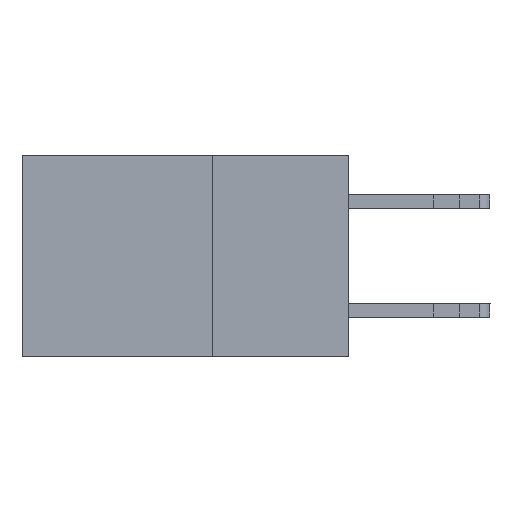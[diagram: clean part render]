
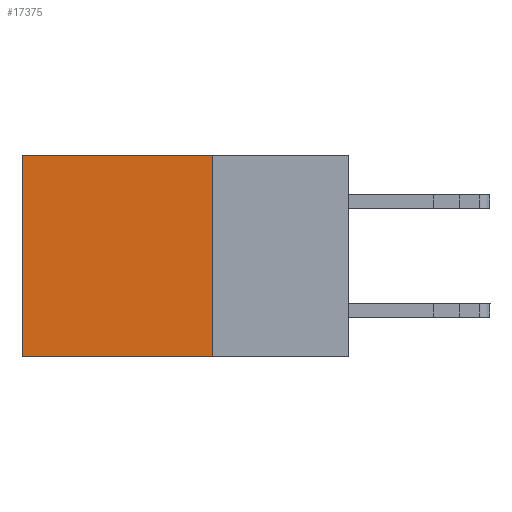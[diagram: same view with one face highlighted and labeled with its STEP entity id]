
A CAD part, left-side view. The second image highlights one B-rep face of the part: STEP entity #17375.
In plain terms, the highlighted planar face has unit normal (-1, 0, 0).
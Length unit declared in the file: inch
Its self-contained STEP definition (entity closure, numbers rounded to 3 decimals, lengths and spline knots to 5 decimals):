
#724 = VECTOR ( 'NONE', #16807, 39.37008 ) ;
#845 = DIRECTION ( 'NONE',  ( 1., 0., 0. ) ) ;
#959 = VERTEX_POINT ( 'NONE', #1659 ) ;
#1659 = CARTESIAN_POINT ( 'NONE',  ( 0.298, 0.25, 0. ) ) ;
#2360 = DIRECTION ( 'NONE',  ( 0., 0., -1. ) ) ;
#2412 = PLANE ( 'NONE',  #18329 ) ;
#2711 = DIRECTION ( 'NONE',  ( 0., 0., -1. ) ) ;
#4101 = DIRECTION ( 'NONE',  ( 0., 1., 0. ) ) ;
#4830 = ORIENTED_EDGE ( 'NONE', *, *, #10977, .T. ) ;
#5261 = CARTESIAN_POINT ( 'NONE',  ( 0.298, 0.25, 0. ) ) ;
#5357 = VECTOR ( 'NONE', #4101, 39.37008 ) ;
#6009 = EDGE_CURVE ( 'NONE', #14056, #12312, #6137, .T. ) ;
#6137 = LINE ( 'NONE', #12407, #724 ) ;
#7092 = ORIENTED_EDGE ( 'NONE', *, *, #12363, .F. ) ;
#8782 = LINE ( 'NONE', #12883, #5357 ) ;
#9106 = ORIENTED_EDGE ( 'NONE', *, *, #16862, .T. ) ;
#10977 = EDGE_CURVE ( 'NONE', #959, #15305, #8782, .T. ) ;
#12312 = VERTEX_POINT ( 'NONE', #12969 ) ;
#12363 = EDGE_CURVE ( 'NONE', #959, #14056, #14022, .T. ) ;
#12383 = CARTESIAN_POINT ( 'NONE',  ( 0.298, 0.6, 0. ) ) ;
#12407 = CARTESIAN_POINT ( 'NONE',  ( 0.298, 0.25, -0.37 ) ) ;
#12883 = CARTESIAN_POINT ( 'NONE',  ( 0.298, 0.25, 0. ) ) ;
#12969 = CARTESIAN_POINT ( 'NONE',  ( 0.298, 0.6, -0.37 ) ) ;
#13318 = VECTOR ( 'NONE', #2711, 39.37008 ) ;
#14022 = LINE ( 'NONE', #16030, #13318 ) ;
#14030 = DIRECTION ( 'NONE',  ( 0., 0., -1. ) ) ;
#14056 = VERTEX_POINT ( 'NONE', #17019 ) ;
#14177 = EDGE_LOOP ( 'NONE', ( #9106, #16224, #7092, #4830 ) ) ;
#14453 = VECTOR ( 'NONE', #2360, 39.37008 ) ;
#15305 = VERTEX_POINT ( 'NONE', #12383 ) ;
#16030 = CARTESIAN_POINT ( 'NONE',  ( 0.298, 0.25, 0. ) ) ;
#16224 = ORIENTED_EDGE ( 'NONE', *, *, #6009, .F. ) ;
#16807 = DIRECTION ( 'NONE',  ( 0., 1., 0. ) ) ;
#16862 = EDGE_CURVE ( 'NONE', #15305, #12312, #17407, .T. ) ;
#16965 = CARTESIAN_POINT ( 'NONE',  ( 0.298, 0.6, 0. ) ) ;
#17019 = CARTESIAN_POINT ( 'NONE',  ( 0.298, 0.25, -0.37 ) ) ;
#17178 = FACE_OUTER_BOUND ( 'NONE', #14177, .T. ) ;
#17375 = ADVANCED_FACE ( 'NONE', ( #17178 ), #2412, .F. ) ;
#17407 = LINE ( 'NONE', #16965, #14453 ) ;
#18329 = AXIS2_PLACEMENT_3D ( 'NONE', #5261, #845, #14030 ) ;
